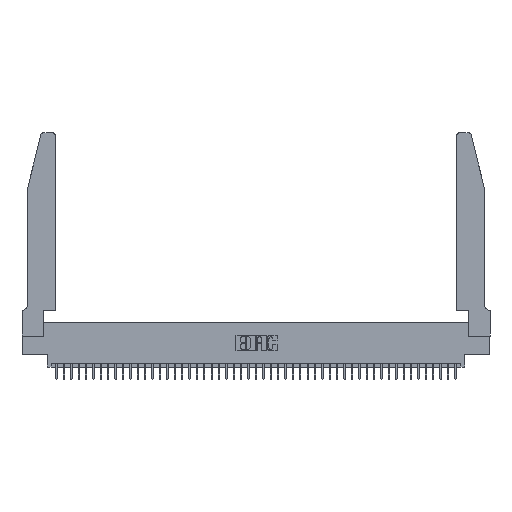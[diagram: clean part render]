
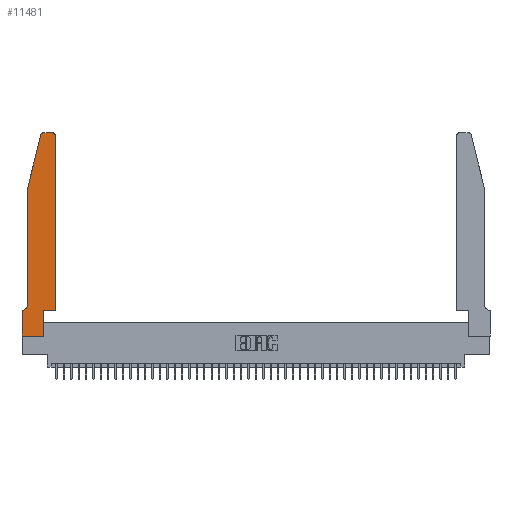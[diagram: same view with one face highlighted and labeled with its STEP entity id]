
A CAD part, top view. The second image highlights one B-rep face of the part: STEP entity #11481.
In plain terms, the highlighted planar face has unit normal (0, 0, 1).
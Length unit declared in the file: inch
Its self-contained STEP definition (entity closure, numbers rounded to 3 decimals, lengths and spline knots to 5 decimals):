
#420 = CARTESIAN_POINT ( 'NONE',  ( 0.4505, 0.35, 0.37 ) ) ;
#720 = CARTESIAN_POINT ( 'NONE',  ( 0.2605, 2.75, 0.37 ) ) ;
#951 = EDGE_LOOP ( 'NONE', ( #38875, #4966, #2337, #25990, #6473, #6805, #23119, #40226, #38314, #38818, #28364, #23880 ) ) ;
#1310 = LINE ( 'NONE', #5408, #35549 ) ;
#1451 = AXIS2_PLACEMENT_3D ( 'NONE', #44596, #11775, #36894 ) ;
#2051 = EDGE_CURVE ( 'NONE', #10245, #23616, #42440, .T. ) ;
#2057 = DIRECTION ( 'NONE',  ( 0., -1., 0. ) ) ;
#2199 = DIRECTION ( 'NONE',  ( 1., 0., 0. ) ) ;
#2243 = EDGE_CURVE ( 'NONE', #6525, #22693, #19436, .T. ) ;
#2337 = ORIENTED_EDGE ( 'NONE', *, *, #17419, .T. ) ;
#2805 = CARTESIAN_POINT ( 'NONE',  ( 0.0755, 2., 0.37 ) ) ;
#3892 = CARTESIAN_POINT ( 'NONE',  ( 0.25487, 2.72718, 0.37 ) ) ;
#4279 = DIRECTION ( 'NONE',  ( -1., 0., 0. ) ) ;
#4673 = EDGE_CURVE ( 'NONE', #23616, #15130, #12043, .T. ) ;
#4966 = ORIENTED_EDGE ( 'NONE', *, *, #29551, .T. ) ;
#5408 = CARTESIAN_POINT ( 'NONE',  ( 0., 0., 0.37 ) ) ;
#6102 = EDGE_CURVE ( 'NONE', #20852, #27488, #1310, .T. ) ;
#6178 = CIRCLE ( 'NONE', #28268, 0.07 ) ;
#6212 = DIRECTION ( 'NONE',  ( 0., -1., 0. ) ) ;
#6473 = ORIENTED_EDGE ( 'NONE', *, *, #22103, .T. ) ;
#6525 = VERTEX_POINT ( 'NONE', #36564 ) ;
#6805 = ORIENTED_EDGE ( 'NONE', *, *, #28924, .T. ) ;
#6877 = VERTEX_POINT ( 'NONE', #3892 ) ;
#7087 = DIRECTION ( 'NONE',  ( 0., 1., 0. ) ) ;
#7833 = DIRECTION ( 'NONE',  ( 0., 0., -1. ) ) ;
#9022 = DIRECTION ( 'NONE',  ( 0., 0., 1. ) ) ;
#9173 = PLANE ( 'NONE',  #43713 ) ;
#10006 = CARTESIAN_POINT ( 'NONE',  ( 0.2865, 0., 0.37 ) ) ;
#10133 = DIRECTION ( 'NONE',  ( -0.239, -0.971, 0. ) ) ;
#10245 = VERTEX_POINT ( 'NONE', #27623 ) ;
#11461 = CARTESIAN_POINT ( 'NONE',  ( 0., 0.35, 0.37 ) ) ;
#11481 = ADVANCED_FACE ( 'NONE', ( #36031 ), #9173, .T. ) ;
#11775 = DIRECTION ( 'NONE',  ( 0., 0., 1. ) ) ;
#12017 = EDGE_CURVE ( 'NONE', #30974, #13061, #37171, .T. ) ;
#12043 = LINE ( 'NONE', #720, #22777 ) ;
#12151 = LINE ( 'NONE', #34489, #15533 ) ;
#12198 = LINE ( 'NONE', #34036, #18376 ) ;
#12940 = DIRECTION ( 'NONE',  ( -1., 0., 0. ) ) ;
#13061 = VERTEX_POINT ( 'NONE', #44300 ) ;
#15130 = VERTEX_POINT ( 'NONE', #30583 ) ;
#15297 = VECTOR ( 'NONE', #19385, 39.37008 ) ;
#15533 = VECTOR ( 'NONE', #2057, 39.37008 ) ;
#16411 = LINE ( 'NONE', #420, #43910 ) ;
#16634 = DIRECTION ( 'NONE',  ( 0., 1., 0. ) ) ;
#17419 = EDGE_CURVE ( 'NONE', #6877, #6525, #21212, .T. ) ;
#18376 = VECTOR ( 'NONE', #34644, 39.37008 ) ;
#18840 = CIRCLE ( 'NONE', #44415, 0.03 ) ;
#19063 = VERTEX_POINT ( 'NONE', #27373 ) ;
#19385 = DIRECTION ( 'NONE',  ( 1., 0., 0. ) ) ;
#19436 = LINE ( 'NONE', #30288, #37882 ) ;
#19737 = DIRECTION ( 'NONE',  ( 1., 0., 0. ) ) ;
#19918 = VERTEX_POINT ( 'NONE', #11461 ) ;
#20139 = CARTESIAN_POINT ( 'NONE',  ( 0.0055, 0.42, 0.37 ) ) ;
#20852 = VERTEX_POINT ( 'NONE', #39934 ) ;
#21212 = LINE ( 'NONE', #2805, #41411 ) ;
#22103 = EDGE_CURVE ( 'NONE', #22693, #19063, #6178, .T. ) ;
#22693 = VERTEX_POINT ( 'NONE', #37165 ) ;
#22746 = EDGE_CURVE ( 'NONE', #19918, #20852, #12151, .T. ) ;
#22777 = VECTOR ( 'NONE', #4279, 39.37008 ) ;
#23119 = ORIENTED_EDGE ( 'NONE', *, *, #22746, .T. ) ;
#23616 = VERTEX_POINT ( 'NONE', #24483 ) ;
#23635 = EDGE_CURVE ( 'NONE', #27488, #30974, #42951, .T. ) ;
#23880 = ORIENTED_EDGE ( 'NONE', *, *, #2051, .T. ) ;
#24483 = CARTESIAN_POINT ( 'NONE',  ( 0.4205, 2.75, 0.37 ) ) ;
#25990 = ORIENTED_EDGE ( 'NONE', *, *, #2243, .T. ) ;
#26790 = DIRECTION ( 'NONE',  ( 1., 0., 0. ) ) ;
#27373 = CARTESIAN_POINT ( 'NONE',  ( 0.0055, 0.35, 0.37 ) ) ;
#27488 = VERTEX_POINT ( 'NONE', #10006 ) ;
#27623 = CARTESIAN_POINT ( 'NONE',  ( 0.4505, 2.72, 0.37 ) ) ;
#28268 = AXIS2_PLACEMENT_3D ( 'NONE', #20139, #7833, #12940 ) ;
#28364 = ORIENTED_EDGE ( 'NONE', *, *, #43998, .T. ) ;
#28394 = VECTOR ( 'NONE', #16634, 39.37008 ) ;
#28924 = EDGE_CURVE ( 'NONE', #19063, #19918, #12198, .T. ) ;
#29551 = EDGE_CURVE ( 'NONE', #15130, #6877, #18840, .T. ) ;
#30288 = CARTESIAN_POINT ( 'NONE',  ( 0.0755, 2., 0.37 ) ) ;
#30373 = CARTESIAN_POINT ( 'NONE',  ( 0.4505, 0.35, 0.37 ) ) ;
#30583 = CARTESIAN_POINT ( 'NONE',  ( 0.284, 2.75, 0.37 ) ) ;
#30974 = VERTEX_POINT ( 'NONE', #34656 ) ;
#33995 = DIRECTION ( 'NONE',  ( 0., 0., 1. ) ) ;
#34036 = CARTESIAN_POINT ( 'NONE',  ( 0.0755, 0.35, 0.37 ) ) ;
#34489 = CARTESIAN_POINT ( 'NONE',  ( 0., 0., 0.37 ) ) ;
#34644 = DIRECTION ( 'NONE',  ( -1., 0., 0. ) ) ;
#34656 = CARTESIAN_POINT ( 'NONE',  ( 0.2865, 0.35, 0.37 ) ) ;
#35549 = VECTOR ( 'NONE', #26790, 39.37008 ) ;
#36031 = FACE_OUTER_BOUND ( 'NONE', #951, .T. ) ;
#36564 = CARTESIAN_POINT ( 'NONE',  ( 0.0755, 2., 0.37 ) ) ;
#36894 = DIRECTION ( 'NONE',  ( 1., 0., 0. ) ) ;
#37165 = CARTESIAN_POINT ( 'NONE',  ( 0.0755, 0.42, 0.37 ) ) ;
#37171 = LINE ( 'NONE', #30373, #15297 ) ;
#37882 = VECTOR ( 'NONE', #6212, 39.37008 ) ;
#38314 = ORIENTED_EDGE ( 'NONE', *, *, #23635, .T. ) ;
#38818 = ORIENTED_EDGE ( 'NONE', *, *, #12017, .T. ) ;
#38875 = ORIENTED_EDGE ( 'NONE', *, *, #4673, .T. ) ;
#39934 = CARTESIAN_POINT ( 'NONE',  ( 0., 0., 0.37 ) ) ;
#40226 = ORIENTED_EDGE ( 'NONE', *, *, #6102, .T. ) ;
#41411 = VECTOR ( 'NONE', #10133, 39.37008 ) ;
#42440 = CIRCLE ( 'NONE', #1451, 0.03 ) ;
#42951 = LINE ( 'NONE', #45783, #28394 ) ;
#43713 = AXIS2_PLACEMENT_3D ( 'NONE', #45448, #9022, #2199 ) ;
#43910 = VECTOR ( 'NONE', #7087, 39.37008 ) ;
#43998 = EDGE_CURVE ( 'NONE', #13061, #10245, #16411, .T. ) ;
#44300 = CARTESIAN_POINT ( 'NONE',  ( 0.4505, 0.35, 0.37 ) ) ;
#44415 = AXIS2_PLACEMENT_3D ( 'NONE', #44665, #33995, #19737 ) ;
#44596 = CARTESIAN_POINT ( 'NONE',  ( 0.4205, 2.72, 0.37 ) ) ;
#44665 = CARTESIAN_POINT ( 'NONE',  ( 0.284, 2.72, 0.37 ) ) ;
#45448 = CARTESIAN_POINT ( 'NONE',  ( 0., 0.35, 0.37 ) ) ;
#45783 = CARTESIAN_POINT ( 'NONE',  ( 0.2865, 0.35, 0.37 ) ) ;
